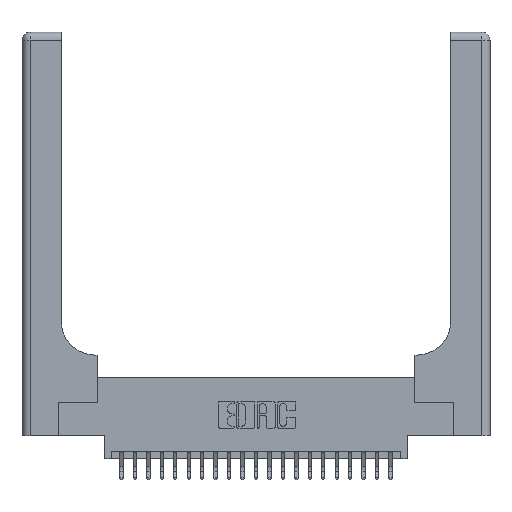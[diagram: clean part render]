
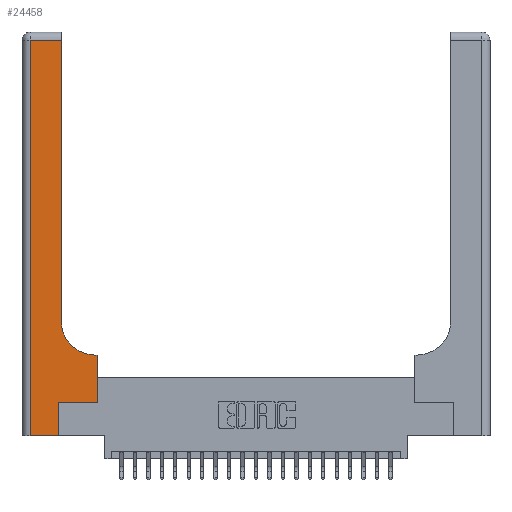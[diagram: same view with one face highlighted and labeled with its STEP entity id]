
A CAD part, top view. The second image highlights one B-rep face of the part: STEP entity #24458.
In plain terms, the highlighted planar face has unit normal (0, 0, 1).
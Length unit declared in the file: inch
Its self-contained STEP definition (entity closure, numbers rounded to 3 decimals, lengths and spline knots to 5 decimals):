
#155 = ORIENTED_EDGE ( 'NONE', *, *, #12232, .T. ) ;
#300 = CARTESIAN_POINT ( 'NONE',  ( 0.5415, 0.6, 0.37 ) ) ;
#745 = EDGE_CURVE ( 'NONE', #19716, #20503, #21333, .T. ) ;
#882 = CARTESIAN_POINT ( 'NONE',  ( 0.269, 0.25, 0.37 ) ) ;
#1076 = DIRECTION ( 'NONE',  ( 0., 1., 0. ) ) ;
#1751 = CARTESIAN_POINT ( 'NONE',  ( 0.06, 2.94, 0.37 ) ) ;
#1833 = VECTOR ( 'NONE', #17294, 39.37008 ) ;
#2296 = LINE ( 'NONE', #23819, #22110 ) ;
#2395 = VECTOR ( 'NONE', #11813, 39.37008 ) ;
#2430 = EDGE_CURVE ( 'NONE', #20503, #2441, #2660, .T. ) ;
#2441 = VERTEX_POINT ( 'NONE', #14518 ) ;
#2458 = CARTESIAN_POINT ( 'NONE',  ( 0., 3., 0.37 ) ) ;
#2589 = VERTEX_POINT ( 'NONE', #1751 ) ;
#2660 = CIRCLE ( 'NONE', #15867, 0.25 ) ;
#2766 = DIRECTION ( 'NONE',  ( 1., 0., 0. ) ) ;
#2914 = FACE_OUTER_BOUND ( 'NONE', #4809, .T. ) ;
#3189 = DIRECTION ( 'NONE',  ( 0., 1., 0. ) ) ;
#3275 = CARTESIAN_POINT ( 'NONE',  ( 0.2915, 3., 0.37 ) ) ;
#3452 = ORIENTED_EDGE ( 'NONE', *, *, #10004, .T. ) ;
#3806 = DIRECTION ( 'NONE',  ( -1., 0., 0. ) ) ;
#3845 = AXIS2_PLACEMENT_3D ( 'NONE', #2458, #6477, #20093 ) ;
#3982 = EDGE_CURVE ( 'NONE', #6734, #2589, #7453, .T. ) ;
#4809 = EDGE_LOOP ( 'NONE', ( #23333, #21357, #20648, #16892, #155, #12254, #3452, #20598, #11710 ) ) ;
#5597 = DIRECTION ( 'NONE',  ( 0., -1., 0. ) ) ;
#6477 = DIRECTION ( 'NONE',  ( 0., 0., -1. ) ) ;
#6734 = VERTEX_POINT ( 'NONE', #16577 ) ;
#7422 = EDGE_CURVE ( 'NONE', #2589, #15576, #19653, .T. ) ;
#7453 = LINE ( 'NONE', #15303, #21579 ) ;
#7891 = VECTOR ( 'NONE', #2766, 39.37008 ) ;
#8316 = CARTESIAN_POINT ( 'NONE',  ( 0.5415, 0.85, 0.37 ) ) ;
#10004 = EDGE_CURVE ( 'NONE', #15768, #19716, #10832, .T. ) ;
#10267 = DIRECTION ( 'NONE',  ( 0., 0., -1. ) ) ;
#10832 = LINE ( 'NONE', #13736, #2395 ) ;
#11710 = ORIENTED_EDGE ( 'NONE', *, *, #2430, .T. ) ;
#11813 = DIRECTION ( 'NONE',  ( 0., 1., 0. ) ) ;
#12024 = DIRECTION ( 'NONE',  ( 1., 0., 0. ) ) ;
#12232 = EDGE_CURVE ( 'NONE', #17302, #22090, #2296, .T. ) ;
#12254 = ORIENTED_EDGE ( 'NONE', *, *, #17414, .T. ) ;
#12396 = DIRECTION ( 'NONE',  ( 1., 0., 0. ) ) ;
#12978 = LINE ( 'NONE', #882, #13893 ) ;
#13736 = CARTESIAN_POINT ( 'NONE',  ( 0.5585, 0.25, 0.37 ) ) ;
#13893 = VECTOR ( 'NONE', #12396, 39.37008 ) ;
#14518 = CARTESIAN_POINT ( 'NONE',  ( 0.2915, 0.85, 0.37 ) ) ;
#14797 = EDGE_CURVE ( 'NONE', #15576, #17302, #17222, .T. ) ;
#15303 = CARTESIAN_POINT ( 'NONE',  ( 0., 2.94, 0.37 ) ) ;
#15559 = LINE ( 'NONE', #3275, #17977 ) ;
#15576 = VERTEX_POINT ( 'NONE', #16773 ) ;
#15768 = VERTEX_POINT ( 'NONE', #21115 ) ;
#15867 = AXIS2_PLACEMENT_3D ( 'NONE', #8316, #10267, #12024 ) ;
#16121 = CARTESIAN_POINT ( 'NONE',  ( 0., 0., 0.37 ) ) ;
#16577 = CARTESIAN_POINT ( 'NONE',  ( 0.2915, 2.94, 0.37 ) ) ;
#16773 = CARTESIAN_POINT ( 'NONE',  ( 0.06, 0., 0.37 ) ) ;
#16892 = ORIENTED_EDGE ( 'NONE', *, *, #14797, .T. ) ;
#17222 = LINE ( 'NONE', #16121, #7891 ) ;
#17294 = DIRECTION ( 'NONE',  ( -1., 0., 0. ) ) ;
#17302 = VERTEX_POINT ( 'NONE', #23473 ) ;
#17414 = EDGE_CURVE ( 'NONE', #22090, #15768, #12978, .T. ) ;
#17675 = PLANE ( 'NONE',  #3845 ) ;
#17977 = VECTOR ( 'NONE', #3189, 39.37008 ) ;
#18814 = CARTESIAN_POINT ( 'NONE',  ( 0.5585, 0.6, 0.37 ) ) ;
#19465 = CARTESIAN_POINT ( 'NONE',  ( 0.2915, 0.6, 0.37 ) ) ;
#19653 = LINE ( 'NONE', #22806, #23549 ) ;
#19716 = VERTEX_POINT ( 'NONE', #18814 ) ;
#20093 = DIRECTION ( 'NONE',  ( -1., 0., 0. ) ) ;
#20503 = VERTEX_POINT ( 'NONE', #300 ) ;
#20545 = CARTESIAN_POINT ( 'NONE',  ( 0.269, 0.25, 0.37 ) ) ;
#20598 = ORIENTED_EDGE ( 'NONE', *, *, #745, .T. ) ;
#20648 = ORIENTED_EDGE ( 'NONE', *, *, #7422, .T. ) ;
#21115 = CARTESIAN_POINT ( 'NONE',  ( 0.5585, 0.25, 0.37 ) ) ;
#21333 = LINE ( 'NONE', #19465, #1833 ) ;
#21357 = ORIENTED_EDGE ( 'NONE', *, *, #3982, .T. ) ;
#21579 = VECTOR ( 'NONE', #3806, 39.37008 ) ;
#22090 = VERTEX_POINT ( 'NONE', #20545 ) ;
#22110 = VECTOR ( 'NONE', #1076, 39.37008 ) ;
#22806 = CARTESIAN_POINT ( 'NONE',  ( 0.06, 3., 0.37 ) ) ;
#23333 = ORIENTED_EDGE ( 'NONE', *, *, #24631, .T. ) ;
#23473 = CARTESIAN_POINT ( 'NONE',  ( 0.269, 0., 0.37 ) ) ;
#23549 = VECTOR ( 'NONE', #5597, 39.37008 ) ;
#23819 = CARTESIAN_POINT ( 'NONE',  ( 0.269, 0., 0.37 ) ) ;
#24458 = ADVANCED_FACE ( 'NONE', ( #2914 ), #17675, .F. ) ;
#24631 = EDGE_CURVE ( 'NONE', #2441, #6734, #15559, .T. ) ;
